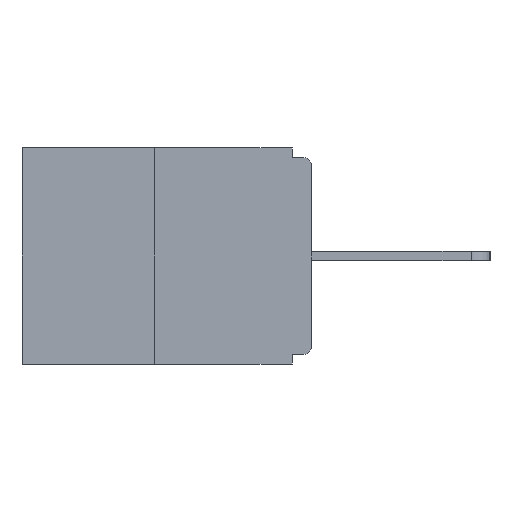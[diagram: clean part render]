
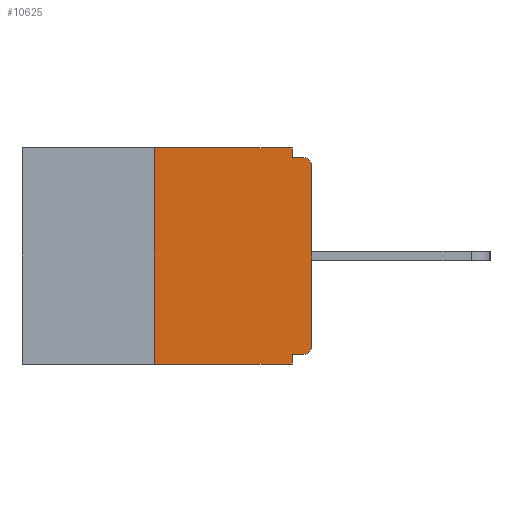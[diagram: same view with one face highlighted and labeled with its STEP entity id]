
A CAD part, left-side view. The second image highlights one B-rep face of the part: STEP entity #10625.
In plain terms, the highlighted planar face has unit normal (-1, 0, 0).
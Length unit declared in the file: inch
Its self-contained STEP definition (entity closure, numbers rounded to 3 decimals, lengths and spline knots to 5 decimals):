
#205 = CARTESIAN_POINT ( 'NONE',  ( 0., 0., -0.313 ) ) ;
#295 = VECTOR ( 'NONE', #9458, 39.37008 ) ;
#522 = DIRECTION ( 'NONE',  ( 0., 0., -1. ) ) ;
#525 = EDGE_CURVE ( 'NONE', #9164, #12204, #15529, .T. ) ;
#735 = CARTESIAN_POINT ( 'NONE',  ( 0., 0.25, -0.343 ) ) ;
#1005 = DIRECTION ( 'NONE',  ( -1., 0., 0. ) ) ;
#1101 = CARTESIAN_POINT ( 'NONE',  ( 0., 0.031, 0. ) ) ;
#2003 = CARTESIAN_POINT ( 'NONE',  ( 0., 0.015, -0.03 ) ) ;
#2017 = VERTEX_POINT ( 'NONE', #3625 ) ;
#2284 = DIRECTION ( 'NONE',  ( 0., 0., -1. ) ) ;
#2456 = ORIENTED_EDGE ( 'NONE', *, *, #17175, .F. ) ;
#2670 = LINE ( 'NONE', #1101, #10340 ) ;
#2686 = VECTOR ( 'NONE', #6775, 39.37008 ) ;
#3210 = LINE ( 'NONE', #13920, #295 ) ;
#3264 = CARTESIAN_POINT ( 'NONE',  ( 0., 0., 0. ) ) ;
#3625 = CARTESIAN_POINT ( 'NONE',  ( 0., 0.031, -0.015 ) ) ;
#3650 = CARTESIAN_POINT ( 'NONE',  ( 0., 0., -0.03 ) ) ;
#3968 = AXIS2_PLACEMENT_3D ( 'NONE', #18451, #1005, #2284 ) ;
#3980 = VERTEX_POINT ( 'NONE', #13539 ) ;
#4032 = AXIS2_PLACEMENT_3D ( 'NONE', #2003, #6499, #522 ) ;
#4155 = ORIENTED_EDGE ( 'NONE', *, *, #9053, .T. ) ;
#4455 = LINE ( 'NONE', #10395, #4856 ) ;
#4637 = CARTESIAN_POINT ( 'NONE',  ( 0., 0.25, 0. ) ) ;
#4856 = VECTOR ( 'NONE', #13216, 39.37008 ) ;
#4948 = VECTOR ( 'NONE', #9218, 39.37008 ) ;
#4992 = ORIENTED_EDGE ( 'NONE', *, *, #6066, .F. ) ;
#5108 = CARTESIAN_POINT ( 'NONE',  ( 0., 0.031, -0.328 ) ) ;
#5174 = VERTEX_POINT ( 'NONE', #13346 ) ;
#5221 = CARTESIAN_POINT ( 'NONE',  ( 0., 0., -0.328 ) ) ;
#5487 = ORIENTED_EDGE ( 'NONE', *, *, #15546, .T. ) ;
#5969 = EDGE_CURVE ( 'NONE', #2017, #12204, #4455, .T. ) ;
#5976 = VECTOR ( 'NONE', #7943, 39.37008 ) ;
#6066 = EDGE_CURVE ( 'NONE', #17626, #12803, #6305, .T. ) ;
#6096 = LINE ( 'NONE', #4637, #10286 ) ;
#6199 = EDGE_CURVE ( 'NONE', #3980, #5174, #8227, .T. ) ;
#6305 = LINE ( 'NONE', #16396, #15108 ) ;
#6499 = DIRECTION ( 'NONE',  ( -1., 0., 0. ) ) ;
#6653 = ORIENTED_EDGE ( 'NONE', *, *, #10702, .F. ) ;
#6775 = DIRECTION ( 'NONE',  ( 0., -1., 0. ) ) ;
#6895 = DIRECTION ( 'NONE',  ( 0., 0., -1. ) ) ;
#7053 = EDGE_LOOP ( 'NONE', ( #15762, #6653, #5487, #4992, #2456, #14727, #4155, #13187, #9784, #8442 ) ) ;
#7524 = EDGE_CURVE ( 'NONE', #12691, #13627, #12362, .T. ) ;
#7943 = DIRECTION ( 'NONE',  ( 0., 1., 0. ) ) ;
#8227 = LINE ( 'NONE', #11244, #2686 ) ;
#8391 = CARTESIAN_POINT ( 'NONE',  ( 0., 0.015, -0.328 ) ) ;
#8442 = ORIENTED_EDGE ( 'NONE', *, *, #18531, .F. ) ;
#9053 = EDGE_CURVE ( 'NONE', #13627, #9164, #16606, .T. ) ;
#9164 = VERTEX_POINT ( 'NONE', #3650 ) ;
#9218 = DIRECTION ( 'NONE',  ( 0., 0., 1. ) ) ;
#9458 = DIRECTION ( 'NONE',  ( 0., -1., 0. ) ) ;
#9503 = LINE ( 'NONE', #5221, #5976 ) ;
#9784 = ORIENTED_EDGE ( 'NONE', *, *, #5969, .F. ) ;
#10268 = CARTESIAN_POINT ( 'NONE',  ( 0., 0.015, -0.015 ) ) ;
#10286 = VECTOR ( 'NONE', #12034, 39.37008 ) ;
#10340 = VECTOR ( 'NONE', #6895, 39.37008 ) ;
#10395 = CARTESIAN_POINT ( 'NONE',  ( 0., 0., -0.015 ) ) ;
#10474 = DIRECTION ( 'NONE',  ( 1., 0., 0. ) ) ;
#10576 = FACE_OUTER_BOUND ( 'NONE', #7053, .T. ) ;
#10625 = ADVANCED_FACE ( 'NONE', ( #10576 ), #17957, .F. ) ;
#10702 = EDGE_CURVE ( 'NONE', #16718, #3980, #6096, .T. ) ;
#11244 = CARTESIAN_POINT ( 'NONE',  ( 0., 0.46, 0. ) ) ;
#12034 = DIRECTION ( 'NONE',  ( 0., 0., 1. ) ) ;
#12204 = VERTEX_POINT ( 'NONE', #10268 ) ;
#12362 = CIRCLE ( 'NONE', #3968, 0.015 ) ;
#12691 = VERTEX_POINT ( 'NONE', #8391 ) ;
#12803 = VERTEX_POINT ( 'NONE', #17534 ) ;
#13187 = ORIENTED_EDGE ( 'NONE', *, *, #525, .T. ) ;
#13216 = DIRECTION ( 'NONE',  ( 0., -1., 0. ) ) ;
#13346 = CARTESIAN_POINT ( 'NONE',  ( 0., 0.031, 0. ) ) ;
#13539 = CARTESIAN_POINT ( 'NONE',  ( 0., 0.25, 0. ) ) ;
#13627 = VERTEX_POINT ( 'NONE', #205 ) ;
#13920 = CARTESIAN_POINT ( 'NONE',  ( 0., 0.46, -0.343 ) ) ;
#14727 = ORIENTED_EDGE ( 'NONE', *, *, #7524, .T. ) ;
#15108 = VECTOR ( 'NONE', #16498, 39.37008 ) ;
#15529 = CIRCLE ( 'NONE', #4032, 0.015 ) ;
#15546 = EDGE_CURVE ( 'NONE', #16718, #12803, #3210, .T. ) ;
#15762 = ORIENTED_EDGE ( 'NONE', *, *, #6199, .F. ) ;
#16174 = AXIS2_PLACEMENT_3D ( 'NONE', #16218, #10474, #16395 ) ;
#16218 = CARTESIAN_POINT ( 'NONE',  ( 0., 0.46, 0. ) ) ;
#16395 = DIRECTION ( 'NONE',  ( 0., 0., -1. ) ) ;
#16396 = CARTESIAN_POINT ( 'NONE',  ( 0., 0.031, -0.343 ) ) ;
#16498 = DIRECTION ( 'NONE',  ( 0., 0., -1. ) ) ;
#16606 = LINE ( 'NONE', #3264, #4948 ) ;
#16718 = VERTEX_POINT ( 'NONE', #735 ) ;
#17175 = EDGE_CURVE ( 'NONE', #12691, #17626, #9503, .T. ) ;
#17534 = CARTESIAN_POINT ( 'NONE',  ( 0., 0.031, -0.343 ) ) ;
#17626 = VERTEX_POINT ( 'NONE', #5108 ) ;
#17957 = PLANE ( 'NONE',  #16174 ) ;
#18451 = CARTESIAN_POINT ( 'NONE',  ( 0., 0.015, -0.313 ) ) ;
#18531 = EDGE_CURVE ( 'NONE', #5174, #2017, #2670, .T. ) ;
